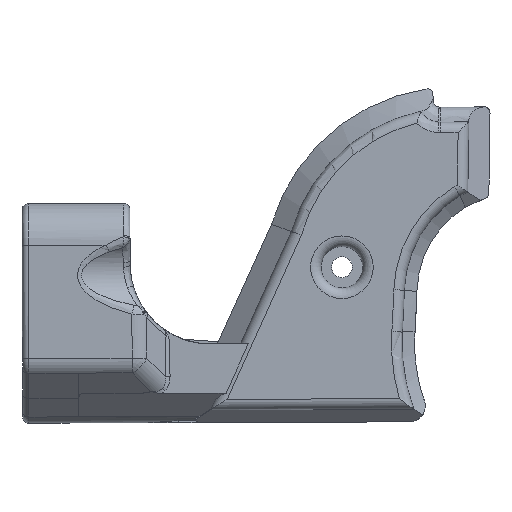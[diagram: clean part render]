
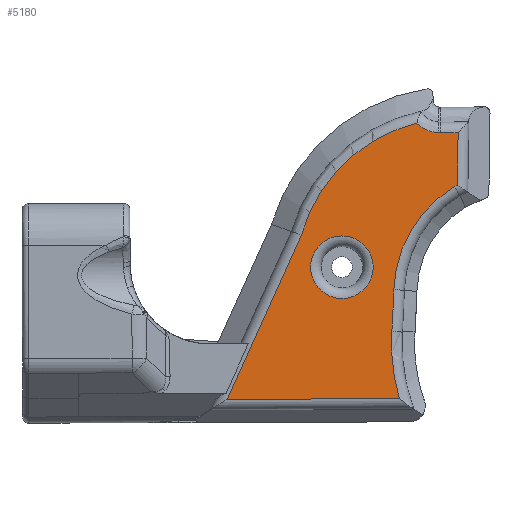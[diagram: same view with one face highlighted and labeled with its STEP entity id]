
A CAD part, left-side view. The second image highlights one B-rep face of the part: STEP entity #5180.
In plain terms, the highlighted planar face has unit normal (-1, 0, 0).
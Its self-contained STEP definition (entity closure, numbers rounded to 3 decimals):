
#86=FACE_BOUND('',#685,.T.);
#127=PLANE('',#5613);
#373=FACE_OUTER_BOUND('',#684,.T.);
#684=EDGE_LOOP('',(#3928,#3929,#3930,#3931,#3932,#3933,#3934,#3935,#3936,
#3937,#3938));
#685=EDGE_LOOP('',(#3939));
#907=CIRCLE('',#5438,349.96);
#969=CIRCLE('',#5610,7.54);
#972=CIRCLE('',#5614,30.086);
#973=CIRCLE('',#5615,38.544);
#974=CIRCLE('',#5616,47.886);
#1155=B_SPLINE_CURVE_WITH_KNOTS('',3,(#11428,#11429,#11430,#11431,#11432),
 .UNSPECIFIED.,.F.,.F.,(4,1,4),(-0.583,-0.335,0.),
 .UNSPECIFIED.);
#1469=LINE('',#10641,#1749);
#1542=LINE('',#11420,#1822);
#1543=LINE('',#11422,#1823);
#1544=LINE('',#11424,#1824);
#1545=LINE('',#11426,#1825);
#1546=LINE('',#11435,#1826);
#1749=VECTOR('',#6214,10.);
#1822=VECTOR('',#6487,10.);
#1823=VECTOR('',#6488,10.);
#1824=VECTOR('',#6489,10.);
#1825=VECTOR('',#6490,10.);
#1826=VECTOR('',#6493,10.);
#2025=VERTEX_POINT('',#10183);
#2028=VERTEX_POINT('',#10188);
#2134=VERTEX_POINT('',#10638);
#2135=VERTEX_POINT('',#10640);
#2204=VERTEX_POINT('',#11411);
#2206=VERTEX_POINT('',#11417);
#2207=VERTEX_POINT('',#11419);
#2208=VERTEX_POINT('',#11421);
#2209=VERTEX_POINT('',#11423);
#2210=VERTEX_POINT('',#11425);
#2211=VERTEX_POINT('',#11427);
#2212=VERTEX_POINT('',#11434);
#2572=EDGE_CURVE('',#2028,#2025,#907,.T.);
#2707=EDGE_CURVE('',#2134,#2135,#1469,.T.);
#2843=EDGE_CURVE('',#2204,#2204,#969,.T.);
#2846=EDGE_CURVE('',#2206,#2028,#972,.T.);
#2847=EDGE_CURVE('',#2207,#2206,#1542,.T.);
#2848=EDGE_CURVE('',#2208,#2207,#1543,.T.);
#2849=EDGE_CURVE('',#2209,#2208,#1544,.T.);
#2850=EDGE_CURVE('',#2210,#2209,#1545,.T.);
#2851=EDGE_CURVE('',#2211,#2210,#1155,.T.);
#2852=EDGE_CURVE('',#2135,#2211,#973,.T.);
#2853=EDGE_CURVE('',#2212,#2134,#1546,.T.);
#2854=EDGE_CURVE('',#2025,#2212,#974,.T.);
#3928=ORIENTED_EDGE('',*,*,#2572,.F.);
#3929=ORIENTED_EDGE('',*,*,#2846,.F.);
#3930=ORIENTED_EDGE('',*,*,#2847,.F.);
#3931=ORIENTED_EDGE('',*,*,#2848,.F.);
#3932=ORIENTED_EDGE('',*,*,#2849,.F.);
#3933=ORIENTED_EDGE('',*,*,#2850,.F.);
#3934=ORIENTED_EDGE('',*,*,#2851,.F.);
#3935=ORIENTED_EDGE('',*,*,#2852,.F.);
#3936=ORIENTED_EDGE('',*,*,#2707,.F.);
#3937=ORIENTED_EDGE('',*,*,#2853,.F.);
#3938=ORIENTED_EDGE('',*,*,#2854,.F.);
#3939=ORIENTED_EDGE('',*,*,#2843,.F.);
#5180=ADVANCED_FACE('',(#373,#86),#127,.F.);
#5438=AXIS2_PLACEMENT_3D('',#10190,#5995,#5996);
#5610=AXIS2_PLACEMENT_3D('',#11412,#6477,#6478);
#5613=AXIS2_PLACEMENT_3D('',#11416,#6483,#6484);
#5614=AXIS2_PLACEMENT_3D('',#11418,#6485,#6486);
#5615=AXIS2_PLACEMENT_3D('',#11433,#6491,#6492);
#5616=AXIS2_PLACEMENT_3D('',#11436,#6494,#6495);
#5995=DIRECTION('center_axis',(1.,0.,0.));
#5996=DIRECTION('ref_axis',(0.,-0.999,-0.046));
#6214=DIRECTION('',(0.,-0.412,0.911));
#6477=DIRECTION('center_axis',(-1.,0.,0.));
#6478=DIRECTION('ref_axis',(0.,0.,
-1.));
#6483=DIRECTION('center_axis',(1.,0.,0.));
#6484=DIRECTION('ref_axis',(0.,1.,0.026));
#6485=DIRECTION('center_axis',(-1.,0.,0.));
#6486=DIRECTION('ref_axis',(0.,0.901,0.434));
#6487=DIRECTION('',(0.,0.915,-0.405));
#6488=DIRECTION('',(0.,0.014,-1.));
#6489=DIRECTION('',(0.,-1.,0.005));
#6490=DIRECTION('',(0.,-1.,-0.026));
#6491=DIRECTION('center_axis',(1.,0.,0.));
#6492=DIRECTION('ref_axis',(0.,0.68,0.733));
#6493=DIRECTION('',(0.,1.,-0.003));
#6494=DIRECTION('center_axis',(-1.,0.,0.));
#6495=DIRECTION('ref_axis',(0.,0.996,-0.086));
#10183=CARTESIAN_POINT('',(14.533,-65.45,16.226));
#10188=CARTESIAN_POINT('',(14.533,-65.912,26.25));
#10190=CARTESIAN_POINT('Origin',(14.533,283.872,37.349));
#10638=CARTESIAN_POINT('',(14.533,-25.748,-0.124));
#10640=CARTESIAN_POINT('',(14.533,-43.628,39.412));
#10641=CARTESIAN_POINT('',(14.533,-43.457,39.036));
#11411=CARTESIAN_POINT('',(14.533,-53.413,39.241));
#11412=CARTESIAN_POINT('Origin',(14.533,-53.413,31.701));
#11416=CARTESIAN_POINT('Origin',(14.533,-53.402,34.294));
#11417=CARTESIAN_POINT('',(14.533,-80.617,51.162));
#11418=CARTESIAN_POINT('Origin',(14.533,-95.982,25.295));
#11419=CARTESIAN_POINT('',(14.533,-81.233,51.434));
#11420=CARTESIAN_POINT('',(14.533,-66.188,44.778));
#11421=CARTESIAN_POINT('',(14.533,-81.411,64.154));
#11422=CARTESIAN_POINT('',(14.533,-81.098,41.857));
#11423=CARTESIAN_POINT('',(14.533,-77.181,64.134));
#11424=CARTESIAN_POINT('',(14.533,-68.632,64.095));
#11425=CARTESIAN_POINT('',(14.533,-76.656,64.148));
#11426=CARTESIAN_POINT('',(14.533,-65.67,64.435));
#11427=CARTESIAN_POINT('',(14.533,-71.439,66.408));
#11428=CARTESIAN_POINT('Ctrl Pts',(14.533,-71.441,66.41));
#11429=CARTESIAN_POINT('Ctrl Pts',(14.533,-72.023,65.823));
#11430=CARTESIAN_POINT('Ctrl Pts',(14.533,-73.61,64.661));
#11431=CARTESIAN_POINT('Ctrl Pts',(14.533,-75.541,64.177));
#11432=CARTESIAN_POINT('Ctrl Pts',(14.533,-76.656,64.148));
#11433=CARTESIAN_POINT('Origin',(14.533,-80.74,29.003));
#11434=CARTESIAN_POINT('',(14.533,-67.252,0.016));
#11435=CARTESIAN_POINT('',(14.533,-37.657,-0.084));
#11436=CARTESIAN_POINT('Origin',(14.533,-113.248,13.336));
